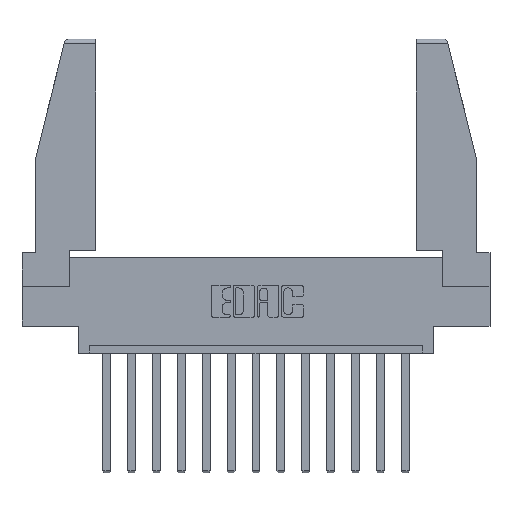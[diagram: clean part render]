
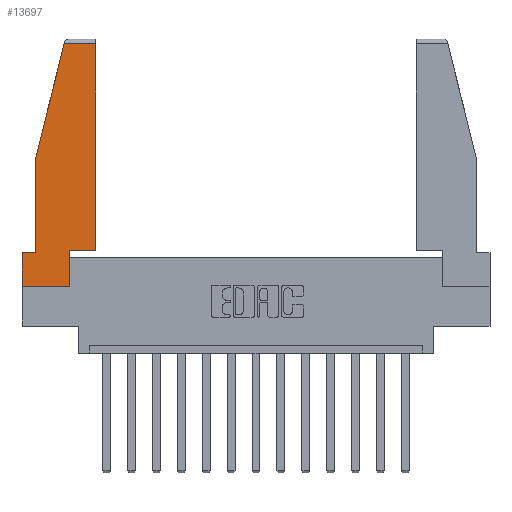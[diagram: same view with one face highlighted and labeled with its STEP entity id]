
A CAD part, top view. The second image highlights one B-rep face of the part: STEP entity #13697.
In plain terms, the highlighted planar face has unit normal (0, 0, 1).
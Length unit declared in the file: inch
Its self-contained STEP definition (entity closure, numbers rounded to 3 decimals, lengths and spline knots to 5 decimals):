
#357 = VERTEX_POINT ( 'NONE', #2616 ) ;
#360 = CARTESIAN_POINT ( 'NONE',  ( 0.086, 0.8, 0. ) ) ;
#660 = DIRECTION ( 'NONE',  ( -1., 0., 0. ) ) ;
#906 = CARTESIAN_POINT ( 'NONE',  ( 0.461, 0.223, 0. ) ) ;
#923 = CARTESIAN_POINT ( 'NONE',  ( 0.297, 0., 0. ) ) ;
#1059 = DIRECTION ( 'NONE',  ( -1., 0., 0. ) ) ;
#1451 = CARTESIAN_POINT ( 'NONE',  ( 0.2636, 1.52, 0. ) ) ;
#1837 = VERTEX_POINT ( 'NONE', #2613 ) ;
#2074 = ORIENTED_EDGE ( 'NONE', *, *, #12067, .T. ) ;
#2114 = FACE_OUTER_BOUND ( 'NONE', #7501, .T. ) ;
#2116 = EDGE_CURVE ( 'NONE', #10328, #10822, #13772, .T. ) ;
#2385 = CARTESIAN_POINT ( 'NONE',  ( 0., 0.21, 0. ) ) ;
#2407 = EDGE_CURVE ( 'NONE', #4997, #357, #7111, .T. ) ;
#2613 = CARTESIAN_POINT ( 'NONE',  ( 0.461, 0.223, 0. ) ) ;
#2616 = CARTESIAN_POINT ( 'NONE',  ( 0.297, 0.223, 0. ) ) ;
#3224 = CARTESIAN_POINT ( 'NONE',  ( 0., 1.52, 0. ) ) ;
#3236 = ORIENTED_EDGE ( 'NONE', *, *, #2116, .T. ) ;
#3454 = CARTESIAN_POINT ( 'NONE',  ( 0.297, 0.223, 0. ) ) ;
#3473 = ORIENTED_EDGE ( 'NONE', *, *, #3625, .T. ) ;
#3625 = EDGE_CURVE ( 'NONE', #12904, #9546, #14690, .T. ) ;
#3749 = VECTOR ( 'NONE', #7228, 39.37008 ) ;
#4568 = EDGE_CURVE ( 'NONE', #9546, #9030, #6294, .T. ) ;
#4588 = EDGE_CURVE ( 'NONE', #10822, #4997, #6676, .T. ) ;
#4949 = VECTOR ( 'NONE', #10217, 39.37008 ) ;
#4997 = VERTEX_POINT ( 'NONE', #7620 ) ;
#5539 = ORIENTED_EDGE ( 'NONE', *, *, #11387, .T. ) ;
#5772 = VECTOR ( 'NONE', #15460, 39.37008 ) ;
#6272 = VECTOR ( 'NONE', #6585, 39.37008 ) ;
#6294 = LINE ( 'NONE', #360, #6272 ) ;
#6346 = ORIENTED_EDGE ( 'NONE', *, *, #11121, .T. ) ;
#6348 = LINE ( 'NONE', #8033, #13938 ) ;
#6448 = ORIENTED_EDGE ( 'NONE', *, *, #4568, .T. ) ;
#6584 = CARTESIAN_POINT ( 'NONE',  ( 0.271, 1.55, 0. ) ) ;
#6585 = DIRECTION ( 'NONE',  ( 0., -1., 0. ) ) ;
#6676 = LINE ( 'NONE', #9227, #4949 ) ;
#7021 = LINE ( 'NONE', #906, #3749 ) ;
#7111 = LINE ( 'NONE', #923, #5772 ) ;
#7228 = DIRECTION ( 'NONE',  ( 0., 1., 0. ) ) ;
#7501 = EDGE_LOOP ( 'NONE', ( #6346, #2074, #3473, #6448, #13111, #3236, #15606, #11249, #5539 ) ) ;
#7620 = CARTESIAN_POINT ( 'NONE',  ( 0.297, 0., 0. ) ) ;
#7667 = CARTESIAN_POINT ( 'NONE',  ( 0., 0.21, 0. ) ) ;
#8033 = CARTESIAN_POINT ( 'NONE',  ( 0., 0.21, 0. ) ) ;
#8400 = CARTESIAN_POINT ( 'NONE',  ( 0., 0., 0. ) ) ;
#9030 = VERTEX_POINT ( 'NONE', #12654 ) ;
#9101 = LINE ( 'NONE', #3224, #14006 ) ;
#9227 = CARTESIAN_POINT ( 'NONE',  ( 0., 0., 0. ) ) ;
#9390 = VECTOR ( 'NONE', #15019, 39.37008 ) ;
#9546 = VERTEX_POINT ( 'NONE', #11236 ) ;
#9677 = DIRECTION ( 'NONE',  ( 1., 0., 0. ) ) ;
#10136 = CARTESIAN_POINT ( 'NONE',  ( 0., 0., 0. ) ) ;
#10170 = DIRECTION ( 'NONE',  ( -0.239, -0.971, 0. ) ) ;
#10217 = DIRECTION ( 'NONE',  ( 1., 0., 0. ) ) ;
#10328 = VERTEX_POINT ( 'NONE', #2385 ) ;
#10438 = VECTOR ( 'NONE', #10170, 39.37008 ) ;
#10822 = VERTEX_POINT ( 'NONE', #10136 ) ;
#11121 = EDGE_CURVE ( 'NONE', #1837, #13438, #7021, .T. ) ;
#11236 = CARTESIAN_POINT ( 'NONE',  ( 0.086, 0.8, 0. ) ) ;
#11249 = ORIENTED_EDGE ( 'NONE', *, *, #2407, .T. ) ;
#11387 = EDGE_CURVE ( 'NONE', #357, #1837, #12882, .T. ) ;
#12067 = EDGE_CURVE ( 'NONE', #13438, #12904, #9101, .T. ) ;
#12077 = DIRECTION ( 'NONE',  ( 1., 0., 0. ) ) ;
#12208 = PLANE ( 'NONE',  #13400 ) ;
#12571 = CARTESIAN_POINT ( 'NONE',  ( 0.461, 1.52, 0. ) ) ;
#12654 = CARTESIAN_POINT ( 'NONE',  ( 0.086, 0.21, 0. ) ) ;
#12882 = LINE ( 'NONE', #3454, #15784 ) ;
#12904 = VERTEX_POINT ( 'NONE', #1451 ) ;
#13111 = ORIENTED_EDGE ( 'NONE', *, *, #13488, .T. ) ;
#13400 = AXIS2_PLACEMENT_3D ( 'NONE', #8400, #14428, #9677 ) ;
#13438 = VERTEX_POINT ( 'NONE', #12571 ) ;
#13488 = EDGE_CURVE ( 'NONE', #9030, #10328, #6348, .T. ) ;
#13697 = ADVANCED_FACE ( 'NONE', ( #2114 ), #12208, .T. ) ;
#13772 = LINE ( 'NONE', #7667, #9390 ) ;
#13938 = VECTOR ( 'NONE', #660, 39.37008 ) ;
#14006 = VECTOR ( 'NONE', #1059, 39.37008 ) ;
#14428 = DIRECTION ( 'NONE',  ( 0., 0., 1. ) ) ;
#14690 = LINE ( 'NONE', #6584, #10438 ) ;
#15019 = DIRECTION ( 'NONE',  ( 0., -1., 0. ) ) ;
#15460 = DIRECTION ( 'NONE',  ( 0., 1., 0. ) ) ;
#15606 = ORIENTED_EDGE ( 'NONE', *, *, #4588, .T. ) ;
#15784 = VECTOR ( 'NONE', #12077, 39.37008 ) ;
